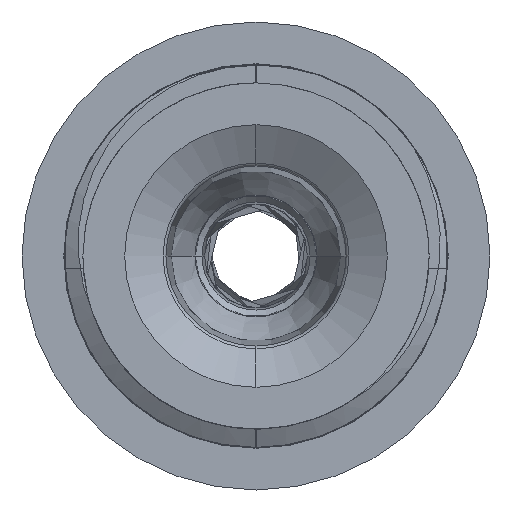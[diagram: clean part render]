
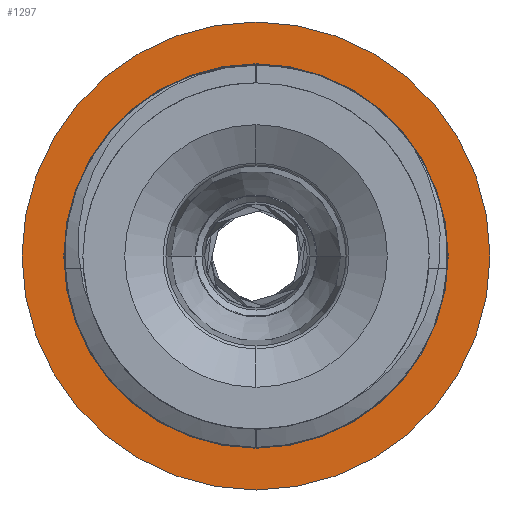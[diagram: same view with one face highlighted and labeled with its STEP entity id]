
A CAD part, left-side view. The second image highlights one B-rep face of the part: STEP entity #1297.
In plain terms, the highlighted planar face has unit normal (-1, 0, 0).
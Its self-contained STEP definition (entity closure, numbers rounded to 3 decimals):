
#431 = PLANE ( 'NONE',  #15827 ) ;
#1114 = CIRCLE ( 'NONE', #4063, 12.446 ) ;
#1297 = ADVANCED_FACE ( 'NONE', ( #14145, #14257 ), #431, .T. ) ;
#1522 = CARTESIAN_POINT ( 'NONE',  ( 0., 0., 0. ) ) ;
#1792 = VERTEX_POINT ( 'NONE', #13182 ) ;
#2673 = ORIENTED_EDGE ( 'NONE', *, *, #20844, .T. ) ;
#3304 = DIRECTION ( 'NONE',  ( 0., 0., 1. ) ) ;
#4063 = AXIS2_PLACEMENT_3D ( 'NONE', #1522, #13843, #10266 ) ;
#5039 = DIRECTION ( 'NONE',  ( 1., 0., 0. ) ) ;
#5497 = CARTESIAN_POINT ( 'NONE',  ( 0., 12.595, -12.595 ) ) ;
#5994 = EDGE_CURVE ( 'NONE', #1792, #6488, #6765, .T. ) ;
#6000 = CARTESIAN_POINT ( 'NONE',  ( 0., 0., 0. ) ) ;
#6488 = VERTEX_POINT ( 'NONE', #10100 ) ;
#6765 = CIRCLE ( 'NONE', #7519, 10.224 ) ;
#6978 = DIRECTION ( 'NONE',  ( 1., 0., 0. ) ) ;
#7426 = EDGE_CURVE ( 'NONE', #16958, #11994, #11524, .T. ) ;
#7519 = AXIS2_PLACEMENT_3D ( 'NONE', #18970, #5039, #11627 ) ;
#7826 = AXIS2_PLACEMENT_3D ( 'NONE', #6000, #9227, #21871 ) ;
#8676 = CARTESIAN_POINT ( 'NONE',  ( 0., 0., 12.446 ) ) ;
#9227 = DIRECTION ( 'NONE',  ( -1., 0., 0. ) ) ;
#9515 = ORIENTED_EDGE ( 'NONE', *, *, #19554, .T. ) ;
#9661 = EDGE_LOOP ( 'NONE', ( #16072, #2673 ) ) ;
#9991 = AXIS2_PLACEMENT_3D ( 'NONE', #11500, #6978, #3304 ) ;
#10041 = CIRCLE ( 'NONE', #9991, 10.224 ) ;
#10100 = CARTESIAN_POINT ( 'NONE',  ( 0., 0., -10.224 ) ) ;
#10266 = DIRECTION ( 'NONE',  ( 0., 0., 1. ) ) ;
#11500 = CARTESIAN_POINT ( 'NONE',  ( 0., 0., 0. ) ) ;
#11524 = CIRCLE ( 'NONE', #7826, 12.446 ) ;
#11627 = DIRECTION ( 'NONE',  ( 0., 0., -1. ) ) ;
#11994 = VERTEX_POINT ( 'NONE', #18262 ) ;
#12538 = DIRECTION ( 'NONE',  ( -1., 0., 0. ) ) ;
#13182 = CARTESIAN_POINT ( 'NONE',  ( 0., 0., 10.224 ) ) ;
#13214 = EDGE_LOOP ( 'NONE', ( #9515, #13443 ) ) ;
#13443 = ORIENTED_EDGE ( 'NONE', *, *, #5994, .T. ) ;
#13843 = DIRECTION ( 'NONE',  ( -1., 0., 0. ) ) ;
#14145 = FACE_OUTER_BOUND ( 'NONE', #9661, .T. ) ;
#14257 = FACE_BOUND ( 'NONE', #13214, .T. ) ;
#15827 = AXIS2_PLACEMENT_3D ( 'NONE', #5497, #12538, #17812 ) ;
#16072 = ORIENTED_EDGE ( 'NONE', *, *, #7426, .T. ) ;
#16958 = VERTEX_POINT ( 'NONE', #8676 ) ;
#17812 = DIRECTION ( 'NONE',  ( 0., 0., 1. ) ) ;
#18262 = CARTESIAN_POINT ( 'NONE',  ( 0., 0., -12.446 ) ) ;
#18970 = CARTESIAN_POINT ( 'NONE',  ( 0., 0., 0. ) ) ;
#19554 = EDGE_CURVE ( 'NONE', #6488, #1792, #10041, .T. ) ;
#20844 = EDGE_CURVE ( 'NONE', #11994, #16958, #1114, .T. ) ;
#21871 = DIRECTION ( 'NONE',  ( 0., 0., 1. ) ) ;
